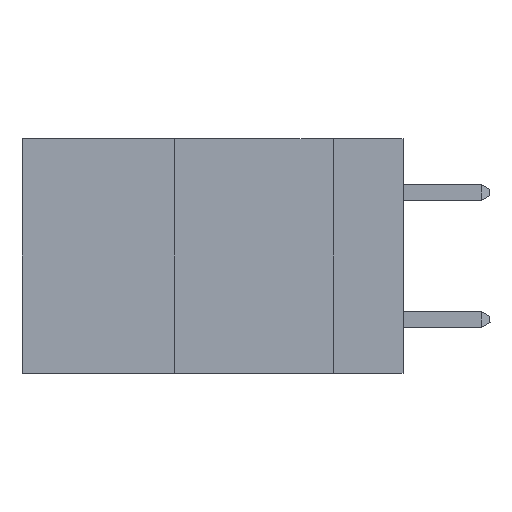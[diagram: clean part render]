
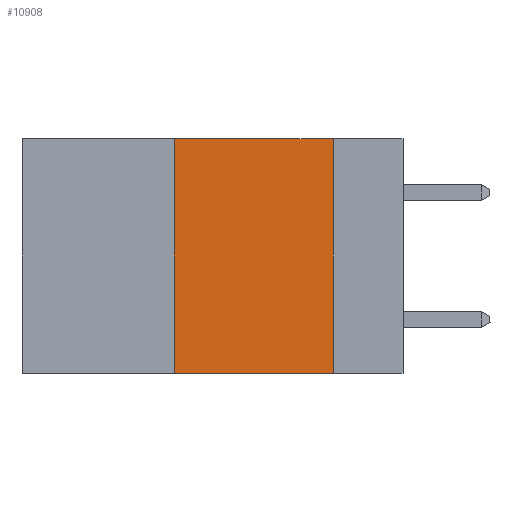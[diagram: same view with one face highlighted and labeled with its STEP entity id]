
A CAD part, left-side view. The second image highlights one B-rep face of the part: STEP entity #10908.
In plain terms, the highlighted planar face has unit normal (-1, 0, 0).
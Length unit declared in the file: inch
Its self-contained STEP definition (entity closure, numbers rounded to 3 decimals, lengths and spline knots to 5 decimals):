
#928 = EDGE_CURVE ( 'NONE', #27968, #943, #11220, .T. ) ;
#943 = VERTEX_POINT ( 'NONE', #20730 ) ;
#1339 = VECTOR ( 'NONE', #21409, 39.37008 ) ;
#3693 = EDGE_CURVE ( 'NONE', #27786, #31605, #6001, .T. ) ;
#3878 = ORIENTED_EDGE ( 'NONE', *, *, #25503, .T. ) ;
#4709 = DIRECTION ( 'NONE',  ( 1., 0., 0. ) ) ;
#4827 = ORIENTED_EDGE ( 'NONE', *, *, #3693, .F. ) ;
#6001 = LINE ( 'NONE', #32511, #31358 ) ;
#7246 = CARTESIAN_POINT ( 'NONE',  ( 0., 0.11, 0. ) ) ;
#7736 = PLANE ( 'NONE',  #26041 ) ;
#8661 = ORIENTED_EDGE ( 'NONE', *, *, #19009, .F. ) ;
#10908 = ADVANCED_FACE ( 'NONE', ( #24792 ), #7736, .F. ) ;
#11220 = LINE ( 'NONE', #29435, #30704 ) ;
#11748 = DIRECTION ( 'NONE',  ( 0., -1., 0. ) ) ;
#14543 = LINE ( 'NONE', #14655, #1339 ) ;
#14655 = CARTESIAN_POINT ( 'NONE',  ( 0., 0.6, -0.37 ) ) ;
#15689 = VECTOR ( 'NONE', #11748, 39.37008 ) ;
#17612 = CARTESIAN_POINT ( 'NONE',  ( 0., 0.36, -0.37 ) ) ;
#19009 = EDGE_CURVE ( 'NONE', #943, #27786, #31743, .T. ) ;
#20730 = CARTESIAN_POINT ( 'NONE',  ( 0., 0.36, 0. ) ) ;
#21409 = DIRECTION ( 'NONE',  ( 0., -1., 0. ) ) ;
#24792 = FACE_OUTER_BOUND ( 'NONE', #34440, .T. ) ;
#25503 = EDGE_CURVE ( 'NONE', #27968, #31605, #14543, .T. ) ;
#26041 = AXIS2_PLACEMENT_3D ( 'NONE', #29494, #4709, #26506 ) ;
#26506 = DIRECTION ( 'NONE',  ( 0., 0., -1. ) ) ;
#27657 = CARTESIAN_POINT ( 'NONE',  ( 0., 0.6, 0. ) ) ;
#27786 = VERTEX_POINT ( 'NONE', #7246 ) ;
#27968 = VERTEX_POINT ( 'NONE', #17612 ) ;
#29435 = CARTESIAN_POINT ( 'NONE',  ( 0., 0.36, 0. ) ) ;
#29494 = CARTESIAN_POINT ( 'NONE',  ( 0., 0.6, 0. ) ) ;
#30704 = VECTOR ( 'NONE', #38827, 39.37008 ) ;
#31358 = VECTOR ( 'NONE', #33591, 39.37008 ) ;
#31605 = VERTEX_POINT ( 'NONE', #39758 ) ;
#31743 = LINE ( 'NONE', #27657, #15689 ) ;
#32511 = CARTESIAN_POINT ( 'NONE',  ( 0., 0.11, 0. ) ) ;
#33591 = DIRECTION ( 'NONE',  ( 0., 0., -1. ) ) ;
#34440 = EDGE_LOOP ( 'NONE', ( #4827, #8661, #37591, #3878 ) ) ;
#37591 = ORIENTED_EDGE ( 'NONE', *, *, #928, .F. ) ;
#38827 = DIRECTION ( 'NONE',  ( 0., 0., 1. ) ) ;
#39758 = CARTESIAN_POINT ( 'NONE',  ( 0., 0.11, -0.37 ) ) ;
